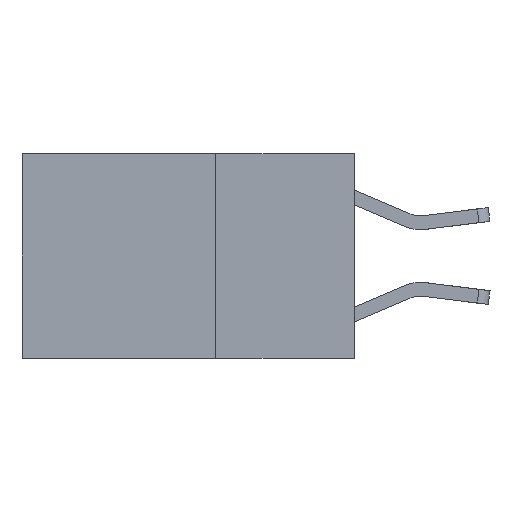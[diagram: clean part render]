
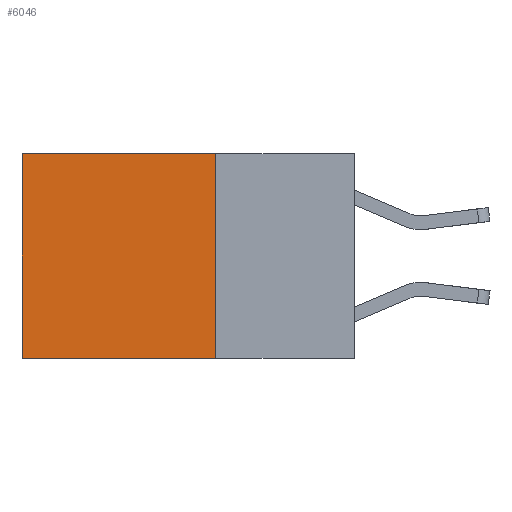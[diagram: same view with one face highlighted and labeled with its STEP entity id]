
A CAD part, left-side view. The second image highlights one B-rep face of the part: STEP entity #6046.
In plain terms, the highlighted planar face has unit normal (-1, 0, 0).
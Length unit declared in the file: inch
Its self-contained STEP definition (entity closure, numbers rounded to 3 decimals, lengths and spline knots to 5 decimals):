
#221 = LINE ( 'NONE', #5176, #2547 ) ;
#318 = CARTESIAN_POINT ( 'NONE',  ( 0.2625, 0.6, -0.37 ) ) ;
#707 = CARTESIAN_POINT ( 'NONE',  ( 0.2625, 0.25, -0.37 ) ) ;
#1254 = LINE ( 'NONE', #9409, #3935 ) ;
#2113 = CARTESIAN_POINT ( 'NONE',  ( 0.2625, 0.25, -0.37 ) ) ;
#2376 = EDGE_CURVE ( 'NONE', #7057, #4760, #6532, .T. ) ;
#2411 = CARTESIAN_POINT ( 'NONE',  ( 0.2625, 0.25, 0. ) ) ;
#2547 = VECTOR ( 'NONE', #7248, 39.37008 ) ;
#2559 = LINE ( 'NONE', #7861, #11606 ) ;
#3920 = DIRECTION ( 'NONE',  ( 0., 1., 0. ) ) ;
#3935 = VECTOR ( 'NONE', #9207, 39.37008 ) ;
#4195 = ORIENTED_EDGE ( 'NONE', *, *, #7264, .T. ) ;
#4760 = VERTEX_POINT ( 'NONE', #318 ) ;
#5176 = CARTESIAN_POINT ( 'NONE',  ( 0.2625, 0.6, 0. ) ) ;
#5265 = DIRECTION ( 'NONE',  ( 0., 0., -1. ) ) ;
#5467 = VERTEX_POINT ( 'NONE', #2411 ) ;
#5554 = AXIS2_PLACEMENT_3D ( 'NONE', #12281, #8238, #5265 ) ;
#5874 = EDGE_LOOP ( 'NONE', ( #4195, #5941, #11778, #6916 ) ) ;
#5941 = ORIENTED_EDGE ( 'NONE', *, *, #2376, .F. ) ;
#6046 = ADVANCED_FACE ( 'NONE', ( #6798 ), #11258, .F. ) ;
#6532 = LINE ( 'NONE', #707, #7894 ) ;
#6798 = FACE_OUTER_BOUND ( 'NONE', #5874, .T. ) ;
#6916 = ORIENTED_EDGE ( 'NONE', *, *, #6980, .T. ) ;
#6980 = EDGE_CURVE ( 'NONE', #5467, #11900, #2559, .T. ) ;
#7057 = VERTEX_POINT ( 'NONE', #2113 ) ;
#7248 = DIRECTION ( 'NONE',  ( 0., 0., -1. ) ) ;
#7264 = EDGE_CURVE ( 'NONE', #11900, #4760, #221, .T. ) ;
#7861 = CARTESIAN_POINT ( 'NONE',  ( 0.2625, 0.25, 0. ) ) ;
#7894 = VECTOR ( 'NONE', #10772, 39.37008 ) ;
#8168 = EDGE_CURVE ( 'NONE', #5467, #7057, #1254, .T. ) ;
#8238 = DIRECTION ( 'NONE',  ( 1., 0., 0. ) ) ;
#8991 = CARTESIAN_POINT ( 'NONE',  ( 0.2625, 0.6, 0. ) ) ;
#9207 = DIRECTION ( 'NONE',  ( 0., 0., -1. ) ) ;
#9409 = CARTESIAN_POINT ( 'NONE',  ( 0.2625, 0.25, 0. ) ) ;
#10772 = DIRECTION ( 'NONE',  ( 0., 1., 0. ) ) ;
#11258 = PLANE ( 'NONE',  #5554 ) ;
#11606 = VECTOR ( 'NONE', #3920, 39.37008 ) ;
#11778 = ORIENTED_EDGE ( 'NONE', *, *, #8168, .F. ) ;
#11900 = VERTEX_POINT ( 'NONE', #8991 ) ;
#12281 = CARTESIAN_POINT ( 'NONE',  ( 0.2625, 0.25, 0. ) ) ;
